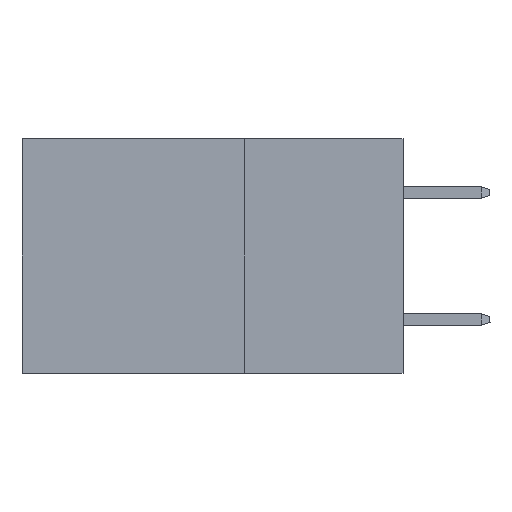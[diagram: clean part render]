
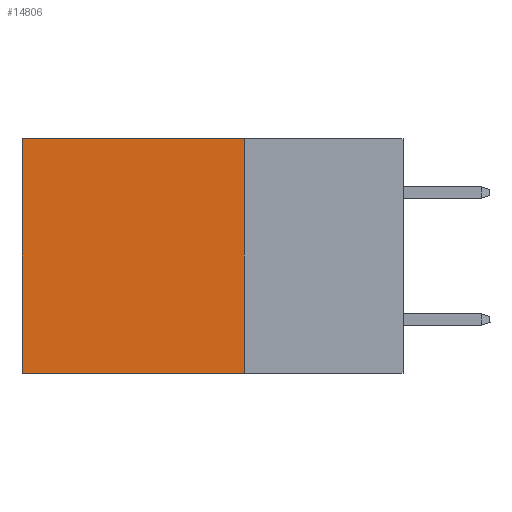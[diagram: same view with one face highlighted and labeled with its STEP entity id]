
A CAD part, left-side view. The second image highlights one B-rep face of the part: STEP entity #14806.
In plain terms, the highlighted planar face has unit normal (-1, 0, 0).
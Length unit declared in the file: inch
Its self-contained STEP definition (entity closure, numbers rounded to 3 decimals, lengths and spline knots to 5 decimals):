
#339 = VECTOR ( 'NONE', #3623, 39.37008 ) ;
#438 = DIRECTION ( 'NONE',  ( 0., 0., -1. ) ) ;
#517 = ORIENTED_EDGE ( 'NONE', *, *, #21642, .T. ) ;
#623 = AXIS2_PLACEMENT_3D ( 'NONE', #13077, #9127, #22497 ) ;
#705 = CARTESIAN_POINT ( 'NONE',  ( 0.2875, 0.6, 0. ) ) ;
#1594 = CARTESIAN_POINT ( 'NONE',  ( 0.2875, 0.25, 0. ) ) ;
#2361 = LINE ( 'NONE', #9921, #18465 ) ;
#3454 = VERTEX_POINT ( 'NONE', #705 ) ;
#3623 = DIRECTION ( 'NONE',  ( 0., 0., -1. ) ) ;
#6620 = VERTEX_POINT ( 'NONE', #15320 ) ;
#7388 = PLANE ( 'NONE',  #623 ) ;
#7848 = VERTEX_POINT ( 'NONE', #1594 ) ;
#8463 = DIRECTION ( 'NONE',  ( 0., 1., 0. ) ) ;
#8892 = EDGE_CURVE ( 'NONE', #3454, #6620, #24448, .T. ) ;
#9127 = DIRECTION ( 'NONE',  ( 1., 0., 0. ) ) ;
#9921 = CARTESIAN_POINT ( 'NONE',  ( 0.2875, 0.25, -0.37 ) ) ;
#10321 = CARTESIAN_POINT ( 'NONE',  ( 0.2875, 0.25, 0. ) ) ;
#10635 = CARTESIAN_POINT ( 'NONE',  ( 0.2875, 0.25, -0.37 ) ) ;
#11074 = VERTEX_POINT ( 'NONE', #10635 ) ;
#11926 = EDGE_LOOP ( 'NONE', ( #13170, #15427, #18615, #517 ) ) ;
#11940 = LINE ( 'NONE', #10321, #13165 ) ;
#13020 = EDGE_CURVE ( 'NONE', #7848, #11074, #17401, .T. ) ;
#13036 = CARTESIAN_POINT ( 'NONE',  ( 0.2875, 0.6, 0. ) ) ;
#13077 = CARTESIAN_POINT ( 'NONE',  ( 0.2875, 0.25, 0. ) ) ;
#13165 = VECTOR ( 'NONE', #8463, 39.37008 ) ;
#13170 = ORIENTED_EDGE ( 'NONE', *, *, #8892, .T. ) ;
#14052 = EDGE_CURVE ( 'NONE', #11074, #6620, #2361, .T. ) ;
#14806 = ADVANCED_FACE ( 'NONE', ( #14933 ), #7388, .F. ) ;
#14933 = FACE_OUTER_BOUND ( 'NONE', #11926, .T. ) ;
#15320 = CARTESIAN_POINT ( 'NONE',  ( 0.2875, 0.6, -0.37 ) ) ;
#15427 = ORIENTED_EDGE ( 'NONE', *, *, #14052, .F. ) ;
#17401 = LINE ( 'NONE', #20877, #19211 ) ;
#17469 = DIRECTION ( 'NONE',  ( 0., 1., 0. ) ) ;
#18465 = VECTOR ( 'NONE', #17469, 39.37008 ) ;
#18615 = ORIENTED_EDGE ( 'NONE', *, *, #13020, .F. ) ;
#19211 = VECTOR ( 'NONE', #438, 39.37008 ) ;
#20877 = CARTESIAN_POINT ( 'NONE',  ( 0.2875, 0.25, 0. ) ) ;
#21642 = EDGE_CURVE ( 'NONE', #7848, #3454, #11940, .T. ) ;
#22497 = DIRECTION ( 'NONE',  ( 0., 0., -1. ) ) ;
#24448 = LINE ( 'NONE', #13036, #339 ) ;
